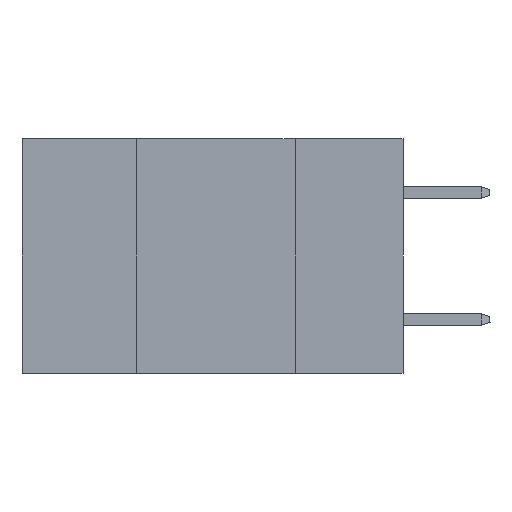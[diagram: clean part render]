
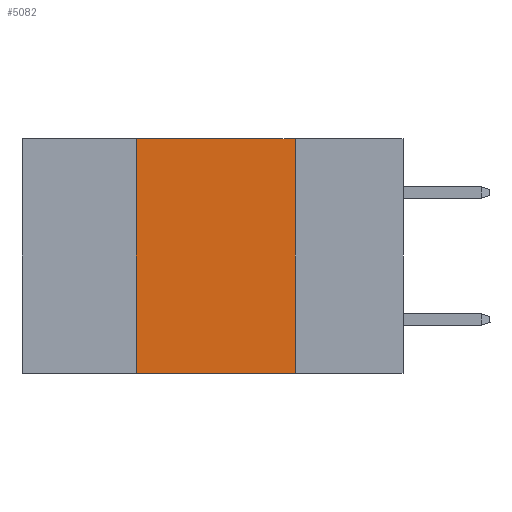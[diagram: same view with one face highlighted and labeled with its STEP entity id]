
A CAD part, left-side view. The second image highlights one B-rep face of the part: STEP entity #5082.
In plain terms, the highlighted planar face has unit normal (-1, 0, 0).
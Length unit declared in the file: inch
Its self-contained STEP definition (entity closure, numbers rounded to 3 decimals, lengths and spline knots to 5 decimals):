
#2126 = VERTEX_POINT ( 'NONE', #28161 ) ;
#4487 = DIRECTION ( 'NONE',  ( 0., -1., 0. ) ) ;
#5082 = ADVANCED_FACE ( 'NONE', ( #18677 ), #5726, .F. ) ;
#5086 = CARTESIAN_POINT ( 'NONE',  ( 0., 0.17, 0. ) ) ;
#5726 = PLANE ( 'NONE',  #8019 ) ;
#6173 = DIRECTION ( 'NONE',  ( 0., -1., 0. ) ) ;
#7158 = LINE ( 'NONE', #16662, #11475 ) ;
#7835 = EDGE_CURVE ( 'NONE', #23463, #19766, #18798, .T. ) ;
#7897 = EDGE_LOOP ( 'NONE', ( #28228, #10311, #24952, #31652 ) ) ;
#8019 = AXIS2_PLACEMENT_3D ( 'NONE', #14554, #24247, #29184 ) ;
#10311 = ORIENTED_EDGE ( 'NONE', *, *, #7835, .F. ) ;
#11475 = VECTOR ( 'NONE', #14363, 39.37008 ) ;
#14363 = DIRECTION ( 'NONE',  ( 0., 0., -1. ) ) ;
#14554 = CARTESIAN_POINT ( 'NONE',  ( 0., 0.6, 0. ) ) ;
#15250 = VECTOR ( 'NONE', #16759, 39.37008 ) ;
#15350 = EDGE_CURVE ( 'NONE', #19766, #2126, #7158, .T. ) ;
#15808 = CARTESIAN_POINT ( 'NONE',  ( 0., 0.42, -0.37 ) ) ;
#16170 = CARTESIAN_POINT ( 'NONE',  ( 0., 0.6, 0. ) ) ;
#16441 = VECTOR ( 'NONE', #6173, 39.37008 ) ;
#16662 = CARTESIAN_POINT ( 'NONE',  ( 0., 0.17, 0. ) ) ;
#16759 = DIRECTION ( 'NONE',  ( 0., 0., 1. ) ) ;
#16800 = CARTESIAN_POINT ( 'NONE',  ( 0., 0.42, 0. ) ) ;
#16950 = VERTEX_POINT ( 'NONE', #15808 ) ;
#18677 = FACE_OUTER_BOUND ( 'NONE', #7897, .T. ) ;
#18798 = LINE ( 'NONE', #16170, #16441 ) ;
#19766 = VERTEX_POINT ( 'NONE', #5086 ) ;
#22228 = EDGE_CURVE ( 'NONE', #16950, #2126, #26965, .T. ) ;
#22523 = CARTESIAN_POINT ( 'NONE',  ( 0., 0.6, -0.37 ) ) ;
#23054 = VECTOR ( 'NONE', #4487, 39.37008 ) ;
#23463 = VERTEX_POINT ( 'NONE', #16800 ) ;
#23869 = EDGE_CURVE ( 'NONE', #16950, #23463, #24492, .T. ) ;
#24247 = DIRECTION ( 'NONE',  ( 1., 0., 0. ) ) ;
#24326 = CARTESIAN_POINT ( 'NONE',  ( 0., 0.42, 0. ) ) ;
#24492 = LINE ( 'NONE', #24326, #15250 ) ;
#24952 = ORIENTED_EDGE ( 'NONE', *, *, #23869, .F. ) ;
#26965 = LINE ( 'NONE', #22523, #23054 ) ;
#28161 = CARTESIAN_POINT ( 'NONE',  ( 0., 0.17, -0.37 ) ) ;
#28228 = ORIENTED_EDGE ( 'NONE', *, *, #15350, .F. ) ;
#29184 = DIRECTION ( 'NONE',  ( 0., 0., -1. ) ) ;
#31652 = ORIENTED_EDGE ( 'NONE', *, *, #22228, .T. ) ;
